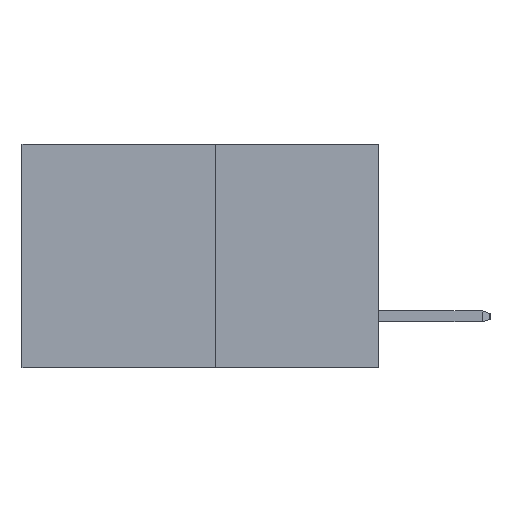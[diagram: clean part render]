
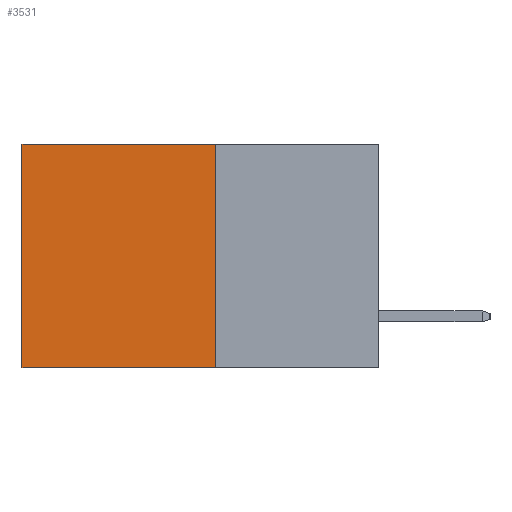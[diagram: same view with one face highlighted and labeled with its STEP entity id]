
A CAD part, left-side view. The second image highlights one B-rep face of the part: STEP entity #3531.
In plain terms, the highlighted planar face has unit normal (-1, 0, 0).
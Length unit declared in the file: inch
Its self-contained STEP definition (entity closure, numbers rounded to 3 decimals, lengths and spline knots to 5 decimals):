
#1857 = CARTESIAN_POINT ( 'NONE',  ( 0.277, 0.59, -0.37 ) ) ;
#2744 = DIRECTION ( 'NONE',  ( 0., 1., 0. ) ) ;
#3445 = ORIENTED_EDGE ( 'NONE', *, *, #13245, .T. ) ;
#3531 = ADVANCED_FACE ( 'NONE', ( #5392 ), #10703, .F. ) ;
#4117 = VECTOR ( 'NONE', #10224, 39.37008 ) ;
#4517 = CARTESIAN_POINT ( 'NONE',  ( 0.277, 0.27, 0. ) ) ;
#4547 = DIRECTION ( 'NONE',  ( 1., 0., 0. ) ) ;
#5365 = EDGE_LOOP ( 'NONE', ( #3445, #19408, #7789, #18201 ) ) ;
#5392 = FACE_OUTER_BOUND ( 'NONE', #5365, .T. ) ;
#7450 = DIRECTION ( 'NONE',  ( 0., 1., 0. ) ) ;
#7789 = ORIENTED_EDGE ( 'NONE', *, *, #11344, .F. ) ;
#8721 = CARTESIAN_POINT ( 'NONE',  ( 0.277, 0.59, -0.37 ) ) ;
#10224 = DIRECTION ( 'NONE',  ( 0., 0., -1. ) ) ;
#10358 = DIRECTION ( 'NONE',  ( 0., 0., -1. ) ) ;
#10566 = CARTESIAN_POINT ( 'NONE',  ( 0.277, 0.27, -0.37 ) ) ;
#10703 = PLANE ( 'NONE',  #12834 ) ;
#11344 = EDGE_CURVE ( 'NONE', #14034, #20380, #15690, .T. ) ;
#12742 = LINE ( 'NONE', #10566, #15989 ) ;
#12834 = AXIS2_PLACEMENT_3D ( 'NONE', #13856, #4547, #15491 ) ;
#13154 = CARTESIAN_POINT ( 'NONE',  ( 0.277, 0.27, -0.37 ) ) ;
#13245 = EDGE_CURVE ( 'NONE', #19283, #15594, #19804, .T. ) ;
#13342 = EDGE_CURVE ( 'NONE', #14034, #19283, #17824, .T. ) ;
#13570 = CARTESIAN_POINT ( 'NONE',  ( 0.277, 0.27, 0. ) ) ;
#13605 = VECTOR ( 'NONE', #7450, 39.37008 ) ;
#13856 = CARTESIAN_POINT ( 'NONE',  ( 0.277, 0.27, -0.37 ) ) ;
#14034 = VERTEX_POINT ( 'NONE', #4517 ) ;
#15048 = CARTESIAN_POINT ( 'NONE',  ( 0.277, 0.27, -0.37 ) ) ;
#15180 = VECTOR ( 'NONE', #10358, 39.37008 ) ;
#15491 = DIRECTION ( 'NONE',  ( 0., 0., -1. ) ) ;
#15594 = VERTEX_POINT ( 'NONE', #1857 ) ;
#15690 = LINE ( 'NONE', #15048, #15180 ) ;
#15989 = VECTOR ( 'NONE', #2744, 39.37008 ) ;
#17694 = CARTESIAN_POINT ( 'NONE',  ( 0.277, 0.59, 0. ) ) ;
#17722 = EDGE_CURVE ( 'NONE', #20380, #15594, #12742, .T. ) ;
#17824 = LINE ( 'NONE', #13570, #13605 ) ;
#18201 = ORIENTED_EDGE ( 'NONE', *, *, #13342, .T. ) ;
#19283 = VERTEX_POINT ( 'NONE', #17694 ) ;
#19408 = ORIENTED_EDGE ( 'NONE', *, *, #17722, .F. ) ;
#19804 = LINE ( 'NONE', #8721, #4117 ) ;
#20380 = VERTEX_POINT ( 'NONE', #13154 ) ;
